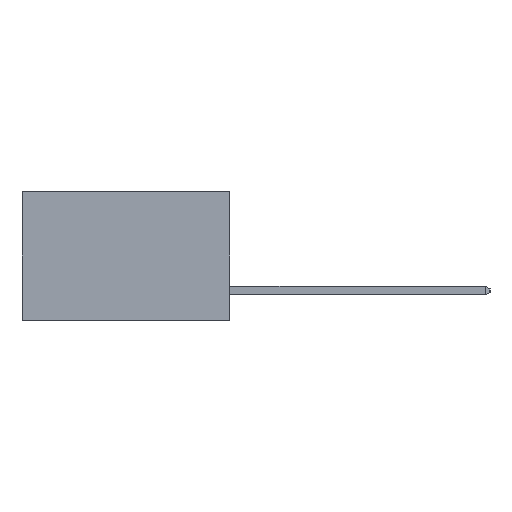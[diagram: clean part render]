
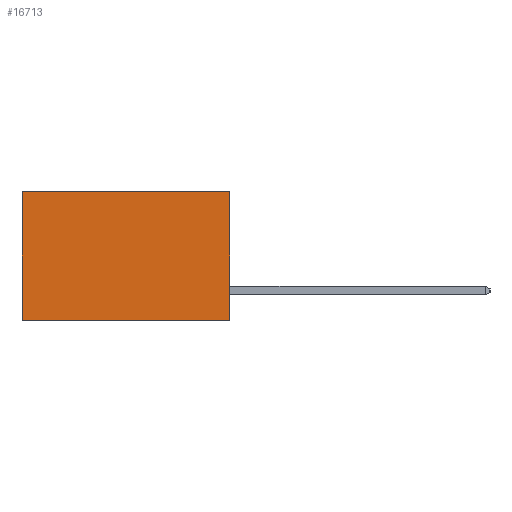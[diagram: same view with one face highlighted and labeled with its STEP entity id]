
A CAD part, left-side view. The second image highlights one B-rep face of the part: STEP entity #16713.
In plain terms, the highlighted planar face has unit normal (-1, 0, 0).
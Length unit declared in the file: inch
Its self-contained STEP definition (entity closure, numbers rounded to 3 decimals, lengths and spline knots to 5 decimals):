
#468 = CARTESIAN_POINT ( 'NONE',  ( 0.298, 0., -0.37 ) ) ;
#1981 = LINE ( 'NONE', #12314, #6785 ) ;
#3048 = VECTOR ( 'NONE', #3858, 39.37008 ) ;
#3858 = DIRECTION ( 'NONE',  ( 0., 0., -1. ) ) ;
#4464 = VERTEX_POINT ( 'NONE', #21827 ) ;
#4788 = ORIENTED_EDGE ( 'NONE', *, *, #9187, .F. ) ;
#5108 = CARTESIAN_POINT ( 'NONE',  ( 0.298, 0., 0. ) ) ;
#6785 = VECTOR ( 'NONE', #8204, 39.37008 ) ;
#7149 = EDGE_CURVE ( 'NONE', #22661, #19595, #9365, .T. ) ;
#8204 = DIRECTION ( 'NONE',  ( 0., 0., -1. ) ) ;
#8661 = CARTESIAN_POINT ( 'NONE',  ( 0.298, 0., -0.37 ) ) ;
#8960 = FACE_OUTER_BOUND ( 'NONE', #17054, .T. ) ;
#8978 = VECTOR ( 'NONE', #14822, 39.37008 ) ;
#9044 = EDGE_CURVE ( 'NONE', #4464, #26218, #1981, .T. ) ;
#9187 = EDGE_CURVE ( 'NONE', #19595, #26218, #18604, .T. ) ;
#9365 = LINE ( 'NONE', #22206, #3048 ) ;
#11353 = DIRECTION ( 'NONE',  ( 0., 0., -1. ) ) ;
#11602 = VECTOR ( 'NONE', #17335, 39.37008 ) ;
#12314 = CARTESIAN_POINT ( 'NONE',  ( 0.298, 0.6, 0. ) ) ;
#13091 = CARTESIAN_POINT ( 'NONE',  ( 0.298, 0., 0. ) ) ;
#13349 = ORIENTED_EDGE ( 'NONE', *, *, #9044, .T. ) ;
#14822 = DIRECTION ( 'NONE',  ( 0., 1., 0. ) ) ;
#16713 = ADVANCED_FACE ( 'NONE', ( #8960 ), #21564, .F. ) ;
#17054 = EDGE_LOOP ( 'NONE', ( #13349, #4788, #20684, #18294 ) ) ;
#17335 = DIRECTION ( 'NONE',  ( 0., 1., 0. ) ) ;
#18294 = ORIENTED_EDGE ( 'NONE', *, *, #25912, .T. ) ;
#18604 = LINE ( 'NONE', #468, #8978 ) ;
#19521 = CARTESIAN_POINT ( 'NONE',  ( 0.298, 0., 0. ) ) ;
#19595 = VERTEX_POINT ( 'NONE', #8661 ) ;
#20684 = ORIENTED_EDGE ( 'NONE', *, *, #7149, .F. ) ;
#21564 = PLANE ( 'NONE',  #24515 ) ;
#21827 = CARTESIAN_POINT ( 'NONE',  ( 0.298, 0.6, 0. ) ) ;
#21845 = LINE ( 'NONE', #5108, #11602 ) ;
#22206 = CARTESIAN_POINT ( 'NONE',  ( 0.298, 0., 0. ) ) ;
#22351 = CARTESIAN_POINT ( 'NONE',  ( 0.298, 0.6, -0.37 ) ) ;
#22661 = VERTEX_POINT ( 'NONE', #13091 ) ;
#23600 = DIRECTION ( 'NONE',  ( 1., 0., 0. ) ) ;
#24515 = AXIS2_PLACEMENT_3D ( 'NONE', #19521, #23600, #11353 ) ;
#25912 = EDGE_CURVE ( 'NONE', #22661, #4464, #21845, .T. ) ;
#26218 = VERTEX_POINT ( 'NONE', #22351 ) ;
